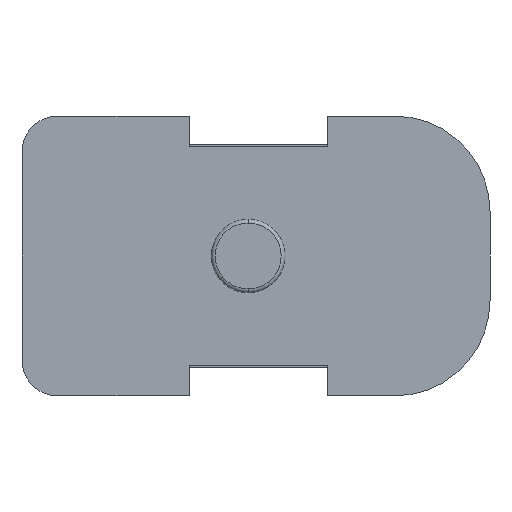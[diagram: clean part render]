
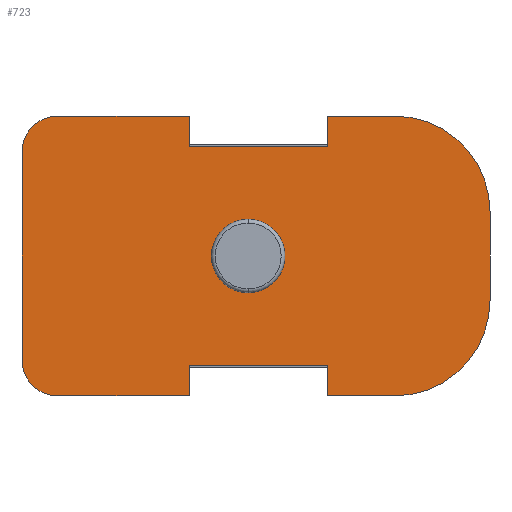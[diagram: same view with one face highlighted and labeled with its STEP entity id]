
A CAD part, front view. The second image highlights one B-rep face of the part: STEP entity #723.
In plain terms, the highlighted planar face has unit normal (0, -1, 0).
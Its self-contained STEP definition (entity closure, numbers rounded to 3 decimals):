
#30 = DIRECTION ( 'NONE',  ( 0., 0., -1. ) ) ;
#36 = CARTESIAN_POINT ( 'NONE',  ( 9.338, 0., -2.946 ) ) ;
#39 = LINE ( 'NONE', #1663, #956 ) ;
#52 = FACE_OUTER_BOUND ( 'NONE', #1445, .T. ) ;
#96 = AXIS2_PLACEMENT_3D ( 'NONE', #998, #286, #990 ) ;
#117 = CARTESIAN_POINT ( 'NONE',  ( -0.384, 0., 0. ) ) ;
#124 = AXIS2_PLACEMENT_3D ( 'NONE', #36, #1064, #1754 ) ;
#135 = ORIENTED_EDGE ( 'NONE', *, *, #240, .T. ) ;
#189 = DIRECTION ( 'NONE',  ( -1., 0., 0. ) ) ;
#191 = VERTEX_POINT ( 'NONE', #1225 ) ;
#208 = CARTESIAN_POINT ( 'NONE',  ( 9.338, 0., 9.296 ) ) ;
#216 = ORIENTED_EDGE ( 'NONE', *, *, #2138, .T. ) ;
#219 = AXIS2_PLACEMENT_3D ( 'NONE', #117, #1329, #294 ) ;
#237 = DIRECTION ( 'NONE',  ( -1., 0., 0. ) ) ;
#240 = EDGE_CURVE ( 'NONE', #2204, #1923, #2228, .T. ) ;
#262 = EDGE_LOOP ( 'NONE', ( #216, #1082 ) ) ;
#270 = CIRCLE ( 'NONE', #124, 6.35 ) ;
#285 = EDGE_CURVE ( 'NONE', #375, #1582, #270, .T. ) ;
#286 = DIRECTION ( 'NONE',  ( 0., 1., 0. ) ) ;
#290 = EDGE_CURVE ( 'NONE', #1143, #375, #1130, .T. ) ;
#291 = ORIENTED_EDGE ( 'NONE', *, *, #819, .T. ) ;
#294 = DIRECTION ( 'NONE',  ( -1., 0., 0. ) ) ;
#298 = VECTOR ( 'NONE', #189, 1000. ) ;
#304 = CARTESIAN_POINT ( 'NONE',  ( -15.414, 0., -6.915 ) ) ;
#313 = ORIENTED_EDGE ( 'NONE', *, *, #285, .T. ) ;
#316 = EDGE_CURVE ( 'NONE', #1891, #1143, #1599, .T. ) ;
#339 = EDGE_CURVE ( 'NONE', #191, #1090, #461, .T. ) ;
#346 = VECTOR ( 'NONE', #472, 1000. ) ;
#349 = LINE ( 'NONE', #2137, #863 ) ;
#356 = EDGE_CURVE ( 'NONE', #1335, #1891, #2207, .T. ) ;
#358 = CARTESIAN_POINT ( 'NONE',  ( -0.886, 0., 0. ) ) ;
#365 = EDGE_CURVE ( 'NONE', #1923, #1335, #349, .T. ) ;
#375 = VERTEX_POINT ( 'NONE', #2176 ) ;
#386 = ORIENTED_EDGE ( 'NONE', *, *, #675, .T. ) ;
#404 = VECTOR ( 'NONE', #939, 1000. ) ;
#448 = CARTESIAN_POINT ( 'NONE',  ( 4.88, 0., 7.29 ) ) ;
#454 = CARTESIAN_POINT ( 'NONE',  ( -2.828, 0., 0. ) ) ;
#461 = CIRCLE ( 'NONE', #96, 2.445 ) ;
#472 = DIRECTION ( 'NONE',  ( -1., 0., 0. ) ) ;
#478 = VECTOR ( 'NONE', #237, 1000. ) ;
#486 = VERTEX_POINT ( 'NONE', #1977 ) ;
#493 = CARTESIAN_POINT ( 'NONE',  ( -4.302, 0., 7.29 ) ) ;
#500 = CIRCLE ( 'NONE', #2168, 6.35 ) ;
#506 = CIRCLE ( 'NONE', #1814, 2.381 ) ;
#533 = LINE ( 'NONE', #1970, #478 ) ;
#609 = DIRECTION ( 'NONE',  ( 0., 0., 1. ) ) ;
#637 = CARTESIAN_POINT ( 'NONE',  ( -13.033, 0., -9.296 ) ) ;
#672 = VECTOR ( 'NONE', #1369, 1000. ) ;
#675 = EDGE_CURVE ( 'NONE', #1868, #2204, #1659, .T. ) ;
#709 = ORIENTED_EDGE ( 'NONE', *, *, #356, .T. ) ;
#723 = ADVANCED_FACE ( 'NONE', ( #52, #971 ), #2088, .F. ) ;
#733 = AXIS2_PLACEMENT_3D ( 'NONE', #358, #1914, #874 ) ;
#755 = VECTOR ( 'NONE', #30, 1000. ) ;
#758 = ORIENTED_EDGE ( 'NONE', *, *, #1917, .T. ) ;
#799 = VERTEX_POINT ( 'NONE', #208 ) ;
#807 = DIRECTION ( 'NONE',  ( 0., -1., 0. ) ) ;
#809 = LINE ( 'NONE', #2028, #346 ) ;
#817 = CARTESIAN_POINT ( 'NONE',  ( 15.688, 0., 2.946 ) ) ;
#819 = EDGE_CURVE ( 'NONE', #890, #1868, #1685, .T. ) ;
#820 = CARTESIAN_POINT ( 'NONE',  ( -4.302, 0., -7.29 ) ) ;
#835 = VECTOR ( 'NONE', #1990, 1000. ) ;
#863 = VECTOR ( 'NONE', #2000, 1000. ) ;
#874 = DIRECTION ( 'NONE',  ( 0., 0., 1. ) ) ;
#890 = VERTEX_POINT ( 'NONE', #1281 ) ;
#897 = EDGE_CURVE ( 'NONE', #799, #1215, #533, .T. ) ;
#939 = DIRECTION ( 'NONE',  ( 1., 0., 0. ) ) ;
#956 = VECTOR ( 'NONE', #609, 1000. ) ;
#959 = CARTESIAN_POINT ( 'NONE',  ( 9.338, 0., 2.946 ) ) ;
#960 = DIRECTION ( 'NONE',  ( 0., 0., -1. ) ) ;
#970 = DIRECTION ( 'NONE',  ( 0., 0., -1. ) ) ;
#971 = FACE_BOUND ( 'NONE', #262, .T. ) ;
#972 = ORIENTED_EDGE ( 'NONE', *, *, #1041, .T. ) ;
#981 = CARTESIAN_POINT ( 'NONE',  ( -4.302, 0., 7.29 ) ) ;
#990 = DIRECTION ( 'NONE',  ( -1., 0., 0. ) ) ;
#998 = CARTESIAN_POINT ( 'NONE',  ( -0.384, 0., 0. ) ) ;
#1030 = DIRECTION ( 'NONE',  ( 0., -1., 0. ) ) ;
#1041 = EDGE_CURVE ( 'NONE', #1582, #2211, #39, .T. ) ;
#1047 = EDGE_CURVE ( 'NONE', #2211, #799, #500, .T. ) ;
#1062 = VERTEX_POINT ( 'NONE', #448 ) ;
#1064 = DIRECTION ( 'NONE',  ( 0., -1., 0. ) ) ;
#1082 = ORIENTED_EDGE ( 'NONE', *, *, #339, .T. ) ;
#1090 = VERTEX_POINT ( 'NONE', #454 ) ;
#1110 = CARTESIAN_POINT ( 'NONE',  ( 15.688, 0., -2.946 ) ) ;
#1130 = LINE ( 'NONE', #1422, #672 ) ;
#1138 = DIRECTION ( 'NONE',  ( 0., 0., -1. ) ) ;
#1143 = VERTEX_POINT ( 'NONE', #1519 ) ;
#1179 = CARTESIAN_POINT ( 'NONE',  ( -13.033, 0., -9.296 ) ) ;
#1215 = VERTEX_POINT ( 'NONE', #2238 ) ;
#1225 = CARTESIAN_POINT ( 'NONE',  ( 2.061, 0., 0. ) ) ;
#1227 = ORIENTED_EDGE ( 'NONE', *, *, #290, .T. ) ;
#1230 = CARTESIAN_POINT ( 'NONE',  ( -4.302, 0., 9.296 ) ) ;
#1281 = CARTESIAN_POINT ( 'NONE',  ( -15.414, 0., 6.915 ) ) ;
#1283 = ORIENTED_EDGE ( 'NONE', *, *, #1047, .T. ) ;
#1309 = VERTEX_POINT ( 'NONE', #493 ) ;
#1329 = DIRECTION ( 'NONE',  ( 0., 1., 0. ) ) ;
#1335 = VERTEX_POINT ( 'NONE', #1878 ) ;
#1339 = DIRECTION ( 'NONE',  ( 0., 0., 1. ) ) ;
#1369 = DIRECTION ( 'NONE',  ( 1., 0., 0. ) ) ;
#1370 = AXIS2_PLACEMENT_3D ( 'NONE', #2073, #1030, #2257 ) ;
#1383 = LINE ( 'NONE', #981, #2254 ) ;
#1404 = CARTESIAN_POINT ( 'NONE',  ( -4.302, 0., -9.296 ) ) ;
#1422 = CARTESIAN_POINT ( 'NONE',  ( 4.88, 0., -9.296 ) ) ;
#1445 = EDGE_LOOP ( 'NONE', ( #313, #972, #1283, #2062, #2232, #1982, #1586, #758, #1568, #291, #386, #135, #1784, #709, #1839, #1227 ) ) ;
#1519 = CARTESIAN_POINT ( 'NONE',  ( 4.88, 0., -9.296 ) ) ;
#1568 = ORIENTED_EDGE ( 'NONE', *, *, #1819, .T. ) ;
#1582 = VERTEX_POINT ( 'NONE', #1110 ) ;
#1586 = ORIENTED_EDGE ( 'NONE', *, *, #1834, .T. ) ;
#1599 = LINE ( 'NONE', #1810, #2002 ) ;
#1654 = CIRCLE ( 'NONE', #219, 2.445 ) ;
#1659 = CIRCLE ( 'NONE', #1370, 2.381 ) ;
#1663 = CARTESIAN_POINT ( 'NONE',  ( 15.688, 0., -2.946 ) ) ;
#1685 = LINE ( 'NONE', #1770, #755 ) ;
#1693 = CARTESIAN_POINT ( 'NONE',  ( 4.88, 0., -7.29 ) ) ;
#1754 = DIRECTION ( 'NONE',  ( -1., 0., 0. ) ) ;
#1761 = EDGE_CURVE ( 'NONE', #1215, #1062, #1886, .T. ) ;
#1770 = CARTESIAN_POINT ( 'NONE',  ( -15.414, 0., 6.915 ) ) ;
#1784 = ORIENTED_EDGE ( 'NONE', *, *, #365, .T. ) ;
#1810 = CARTESIAN_POINT ( 'NONE',  ( 4.88, 0., -7.29 ) ) ;
#1814 = AXIS2_PLACEMENT_3D ( 'NONE', #1842, #807, #2024 ) ;
#1819 = EDGE_CURVE ( 'NONE', #486, #890, #506, .T. ) ;
#1834 = EDGE_CURVE ( 'NONE', #1309, #1949, #1383, .T. ) ;
#1839 = ORIENTED_EDGE ( 'NONE', *, *, #316, .T. ) ;
#1842 = CARTESIAN_POINT ( 'NONE',  ( -13.033, 0., 6.915 ) ) ;
#1868 = VERTEX_POINT ( 'NONE', #304 ) ;
#1872 = EDGE_CURVE ( 'NONE', #1062, #1309, #809, .T. ) ;
#1878 = CARTESIAN_POINT ( 'NONE',  ( -4.302, 0., -7.29 ) ) ;
#1886 = LINE ( 'NONE', #2016, #1941 ) ;
#1891 = VERTEX_POINT ( 'NONE', #1693 ) ;
#1914 = DIRECTION ( 'NONE',  ( 0., 1., 0. ) ) ;
#1917 = EDGE_CURVE ( 'NONE', #1949, #486, #2031, .T. ) ;
#1923 = VERTEX_POINT ( 'NONE', #1404 ) ;
#1925 = CARTESIAN_POINT ( 'NONE',  ( -4.302, 0., 9.296 ) ) ;
#1941 = VECTOR ( 'NONE', #970, 1000. ) ;
#1949 = VERTEX_POINT ( 'NONE', #1925 ) ;
#1970 = CARTESIAN_POINT ( 'NONE',  ( 9.338, 0., 9.296 ) ) ;
#1977 = CARTESIAN_POINT ( 'NONE',  ( -13.033, 0., 9.296 ) ) ;
#1982 = ORIENTED_EDGE ( 'NONE', *, *, #1872, .T. ) ;
#1990 = DIRECTION ( 'NONE',  ( 1., 0., 0. ) ) ;
#2000 = DIRECTION ( 'NONE',  ( 0., 0., 1. ) ) ;
#2002 = VECTOR ( 'NONE', #960, 1000. ) ;
#2016 = CARTESIAN_POINT ( 'NONE',  ( 4.88, 0., 9.296 ) ) ;
#2024 = DIRECTION ( 'NONE',  ( 1., 0., 0. ) ) ;
#2028 = CARTESIAN_POINT ( 'NONE',  ( 4.88, 0., 7.29 ) ) ;
#2031 = LINE ( 'NONE', #1230, #298 ) ;
#2062 = ORIENTED_EDGE ( 'NONE', *, *, #897, .T. ) ;
#2073 = CARTESIAN_POINT ( 'NONE',  ( -13.033, 0., -6.915 ) ) ;
#2088 = PLANE ( 'NONE',  #733 ) ;
#2137 = CARTESIAN_POINT ( 'NONE',  ( -4.302, 0., -9.296 ) ) ;
#2138 = EDGE_CURVE ( 'NONE', #1090, #191, #1654, .T. ) ;
#2168 = AXIS2_PLACEMENT_3D ( 'NONE', #959, #2187, #1138 ) ;
#2176 = CARTESIAN_POINT ( 'NONE',  ( 9.338, 0., -9.296 ) ) ;
#2187 = DIRECTION ( 'NONE',  ( 0., -1., 0. ) ) ;
#2204 = VERTEX_POINT ( 'NONE', #637 ) ;
#2207 = LINE ( 'NONE', #820, #404 ) ;
#2211 = VERTEX_POINT ( 'NONE', #817 ) ;
#2228 = LINE ( 'NONE', #1179, #835 ) ;
#2232 = ORIENTED_EDGE ( 'NONE', *, *, #1761, .T. ) ;
#2238 = CARTESIAN_POINT ( 'NONE',  ( 4.88, 0., 9.296 ) ) ;
#2254 = VECTOR ( 'NONE', #1339, 1000. ) ;
#2257 = DIRECTION ( 'NONE',  ( 0., 0., 1. ) ) ;
